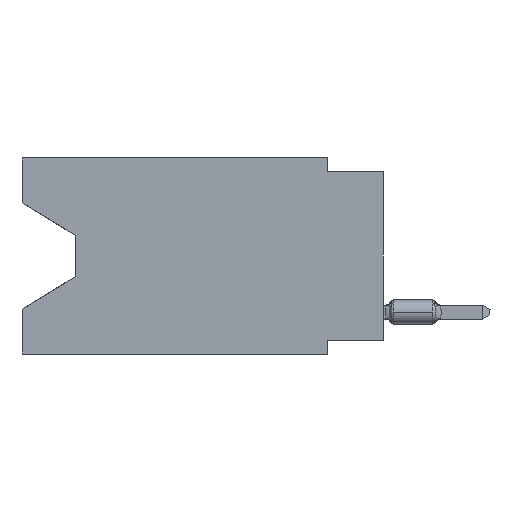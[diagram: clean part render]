
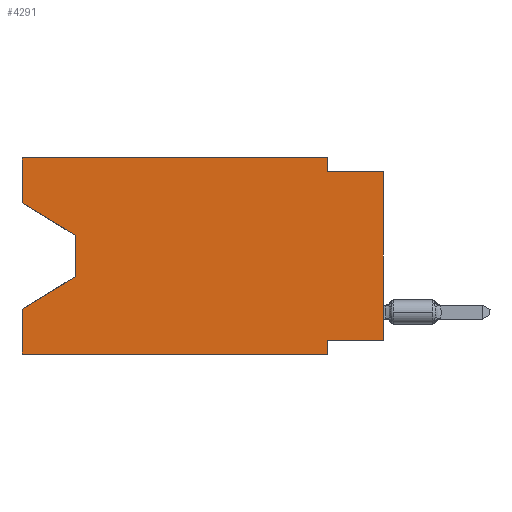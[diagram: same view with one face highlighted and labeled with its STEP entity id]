
A CAD part, left-side view. The second image highlights one B-rep face of the part: STEP entity #4291.
In plain terms, the highlighted planar face has unit normal (-1, 0, 0).
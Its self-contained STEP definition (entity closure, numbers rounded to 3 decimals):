
#15 = CARTESIAN_POINT ( 'NONE',  ( 0., 2.54, -8.89 ) ) ;
#373 = LINE ( 'NONE', #3301, #5807 ) ;
#838 = ORIENTED_EDGE ( 'NONE', *, *, #22129, .F. ) ;
#1145 = CARTESIAN_POINT ( 'NONE',  ( 0., 16.383, -6.852 ) ) ;
#1223 = LINE ( 'NONE', #3386, #24411 ) ;
#1483 = DIRECTION ( 'NONE',  ( 0., -1., 0. ) ) ;
#1786 = CARTESIAN_POINT ( 'NONE',  ( 0., 2.54, -8.89 ) ) ;
#1808 = ORIENTED_EDGE ( 'NONE', *, *, #24311, .T. ) ;
#1934 = CARTESIAN_POINT ( 'NONE',  ( 0., 16.383, 0. ) ) ;
#2016 = VECTOR ( 'NONE', #26536, 1000. ) ;
#2980 = CARTESIAN_POINT ( 'NONE',  ( 0., 13.97, -5.385 ) ) ;
#3070 = EDGE_CURVE ( 'NONE', #17601, #25722, #14221, .T. ) ;
#3154 = ORIENTED_EDGE ( 'NONE', *, *, #3070, .F. ) ;
#3301 = CARTESIAN_POINT ( 'NONE',  ( 0., 16.383, -2.038 ) ) ;
#3386 = CARTESIAN_POINT ( 'NONE',  ( 0., 16.383, -8.89 ) ) ;
#3421 = EDGE_CURVE ( 'NONE', #28838, #29619, #6398, .T. ) ;
#3737 = CARTESIAN_POINT ( 'NONE',  ( 0., 0., -8.255 ) ) ;
#3990 = DIRECTION ( 'NONE',  ( 0., 0., -1. ) ) ;
#4073 = CARTESIAN_POINT ( 'NONE',  ( 0., 16.383, -8.89 ) ) ;
#4291 = ADVANCED_FACE ( 'NONE', ( #25012 ), #17928, .F. ) ;
#5156 = DIRECTION ( 'NONE',  ( 0., 0.855, -0.519 ) ) ;
#5312 = VECTOR ( 'NONE', #5156, 1000. ) ;
#5807 = VECTOR ( 'NONE', #17510, 1000. ) ;
#6183 = DIRECTION ( 'NONE',  ( 1., 0., 0. ) ) ;
#6335 = DIRECTION ( 'NONE',  ( 0., 0., -1. ) ) ;
#6398 = LINE ( 'NONE', #15974, #25807 ) ;
#6686 = DIRECTION ( 'NONE',  ( 0., 1., 0. ) ) ;
#6692 = DIRECTION ( 'NONE',  ( 0., 0., -1. ) ) ;
#6726 = CARTESIAN_POINT ( 'NONE',  ( 0., 0., -0.635 ) ) ;
#6732 = ORIENTED_EDGE ( 'NONE', *, *, #15234, .T. ) ;
#6757 = CARTESIAN_POINT ( 'NONE',  ( 0., 2.54, -0.635 ) ) ;
#7465 = VERTEX_POINT ( 'NONE', #10483 ) ;
#7567 = CARTESIAN_POINT ( 'NONE',  ( 0., 0., -0.635 ) ) ;
#9296 = VERTEX_POINT ( 'NONE', #20866 ) ;
#9441 = DIRECTION ( 'NONE',  ( 0., 0., -1. ) ) ;
#9513 = DIRECTION ( 'NONE',  ( 0., 0., 1. ) ) ;
#10076 = EDGE_CURVE ( 'NONE', #29619, #22473, #18026, .T. ) ;
#10157 = CARTESIAN_POINT ( 'NONE',  ( 0., 16.383, -2.038 ) ) ;
#10483 = CARTESIAN_POINT ( 'NONE',  ( 0., 13.97, -3.505 ) ) ;
#11590 = VECTOR ( 'NONE', #20015, 1000. ) ;
#11598 = ORIENTED_EDGE ( 'NONE', *, *, #11985, .F. ) ;
#11681 = CARTESIAN_POINT ( 'NONE',  ( 0., 16.383, 0. ) ) ;
#11808 = VERTEX_POINT ( 'NONE', #4073 ) ;
#11985 = EDGE_CURVE ( 'NONE', #30233, #17601, #28282, .T. ) ;
#12020 = ORIENTED_EDGE ( 'NONE', *, *, #25199, .F. ) ;
#12738 = LINE ( 'NONE', #14738, #5312 ) ;
#12776 = LINE ( 'NONE', #20164, #11590 ) ;
#13045 = EDGE_LOOP ( 'NONE', ( #29364, #6732, #1808, #12020, #15559, #3154, #11598, #28260, #30083, #30162, #19972, #838 ) ) ;
#13149 = EDGE_CURVE ( 'NONE', #30233, #22473, #12776, .T. ) ;
#13825 = VECTOR ( 'NONE', #6686, 1000. ) ;
#13914 = EDGE_CURVE ( 'NONE', #11808, #25722, #1223, .T. ) ;
#14143 = VERTEX_POINT ( 'NONE', #10157 ) ;
#14221 = LINE ( 'NONE', #15, #28259 ) ;
#14470 = CARTESIAN_POINT ( 'NONE',  ( 0., 2.54, -8.255 ) ) ;
#14738 = CARTESIAN_POINT ( 'NONE',  ( 0., 13.97, -5.385 ) ) ;
#15234 = EDGE_CURVE ( 'NONE', #7465, #20872, #15737, .T. ) ;
#15436 = DIRECTION ( 'NONE',  ( 0., -1., 0. ) ) ;
#15559 = ORIENTED_EDGE ( 'NONE', *, *, #13914, .T. ) ;
#15737 = LINE ( 'NONE', #25126, #16589 ) ;
#15974 = CARTESIAN_POINT ( 'NONE',  ( 0., 2.54, 0. ) ) ;
#16589 = VECTOR ( 'NONE', #3990, 1000. ) ;
#16760 = LINE ( 'NONE', #11681, #30421 ) ;
#16836 = LINE ( 'NONE', #19453, #2016 ) ;
#17510 = DIRECTION ( 'NONE',  ( 0., -0.855, -0.519 ) ) ;
#17601 = VERTEX_POINT ( 'NONE', #14470 ) ;
#17928 = PLANE ( 'NONE',  #28737 ) ;
#17965 = EDGE_CURVE ( 'NONE', #9296, #28838, #22626, .T. ) ;
#18026 = LINE ( 'NONE', #6726, #27721 ) ;
#18193 = EDGE_CURVE ( 'NONE', #14143, #7465, #373, .T. ) ;
#18377 = CARTESIAN_POINT ( 'NONE',  ( 0., 16.383, 0. ) ) ;
#19453 = CARTESIAN_POINT ( 'NONE',  ( 0., 16.383, 0. ) ) ;
#19972 = ORIENTED_EDGE ( 'NONE', *, *, #17965, .F. ) ;
#20015 = DIRECTION ( 'NONE',  ( 0., 0., 1. ) ) ;
#20164 = CARTESIAN_POINT ( 'NONE',  ( 0., 0., 0. ) ) ;
#20866 = CARTESIAN_POINT ( 'NONE',  ( 0., 16.383, 0. ) ) ;
#20872 = VERTEX_POINT ( 'NONE', #2980 ) ;
#22129 = EDGE_CURVE ( 'NONE', #14143, #9296, #16760, .T. ) ;
#22473 = VERTEX_POINT ( 'NONE', #7567 ) ;
#22626 = LINE ( 'NONE', #1934, #23105 ) ;
#22653 = DIRECTION ( 'NONE',  ( 0., -1., 0. ) ) ;
#23105 = VECTOR ( 'NONE', #1483, 1000. ) ;
#24311 = EDGE_CURVE ( 'NONE', #20872, #24514, #12738, .T. ) ;
#24411 = VECTOR ( 'NONE', #15436, 1000. ) ;
#24514 = VERTEX_POINT ( 'NONE', #1145 ) ;
#25012 = FACE_OUTER_BOUND ( 'NONE', #13045, .T. ) ;
#25126 = CARTESIAN_POINT ( 'NONE',  ( 0., 13.97, -3.505 ) ) ;
#25199 = EDGE_CURVE ( 'NONE', #11808, #24514, #16836, .T. ) ;
#25510 = CARTESIAN_POINT ( 'NONE',  ( 0., 0., -8.255 ) ) ;
#25722 = VERTEX_POINT ( 'NONE', #1786 ) ;
#25807 = VECTOR ( 'NONE', #6692, 1000. ) ;
#26536 = DIRECTION ( 'NONE',  ( 0., 0., 1. ) ) ;
#27675 = CARTESIAN_POINT ( 'NONE',  ( 0., 2.54, 0. ) ) ;
#27721 = VECTOR ( 'NONE', #22653, 1000. ) ;
#28259 = VECTOR ( 'NONE', #9441, 1000. ) ;
#28260 = ORIENTED_EDGE ( 'NONE', *, *, #13149, .T. ) ;
#28282 = LINE ( 'NONE', #25510, #13825 ) ;
#28737 = AXIS2_PLACEMENT_3D ( 'NONE', #18377, #6183, #6335 ) ;
#28838 = VERTEX_POINT ( 'NONE', #27675 ) ;
#29364 = ORIENTED_EDGE ( 'NONE', *, *, #18193, .T. ) ;
#29619 = VERTEX_POINT ( 'NONE', #6757 ) ;
#30083 = ORIENTED_EDGE ( 'NONE', *, *, #10076, .F. ) ;
#30162 = ORIENTED_EDGE ( 'NONE', *, *, #3421, .F. ) ;
#30233 = VERTEX_POINT ( 'NONE', #3737 ) ;
#30421 = VECTOR ( 'NONE', #9513, 1000. ) ;
